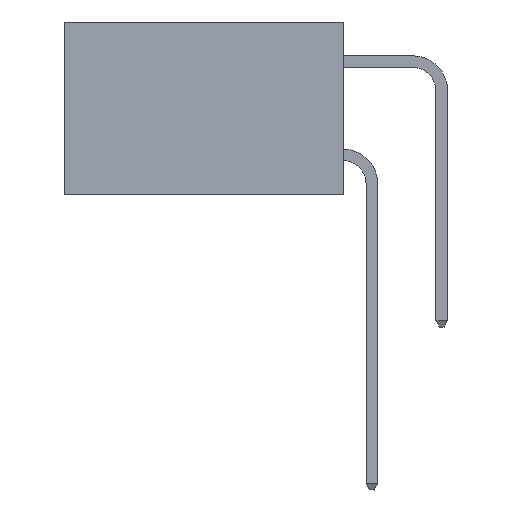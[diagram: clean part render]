
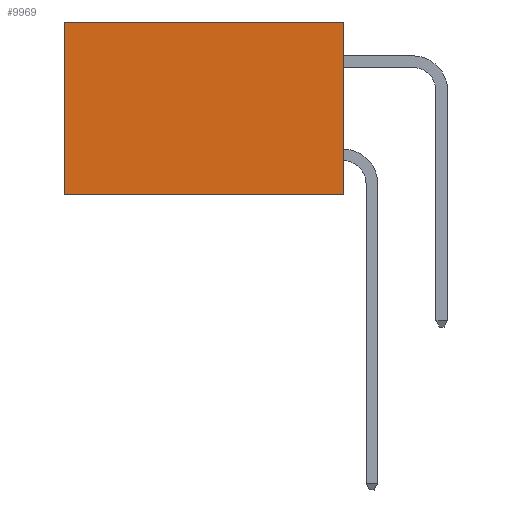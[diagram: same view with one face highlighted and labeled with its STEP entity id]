
A CAD part, left-side view. The second image highlights one B-rep face of the part: STEP entity #9969.
In plain terms, the highlighted planar face has unit normal (-1, 0, 0).
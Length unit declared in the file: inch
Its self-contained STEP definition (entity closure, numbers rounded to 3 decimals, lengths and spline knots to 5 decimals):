
#411 = CARTESIAN_POINT ( 'NONE',  ( 0.298, 0., 0. ) ) ;
#684 = CARTESIAN_POINT ( 'NONE',  ( 0.298, 0., -0.37 ) ) ;
#968 = CARTESIAN_POINT ( 'NONE',  ( 0.298, 0., 0. ) ) ;
#1113 = LINE ( 'NONE', #684, #7513 ) ;
#1353 = ORIENTED_EDGE ( 'NONE', *, *, #10987, .F. ) ;
#1710 = DIRECTION ( 'NONE',  ( 0., 0., -1. ) ) ;
#2029 = ORIENTED_EDGE ( 'NONE', *, *, #10801, .F. ) ;
#2279 = EDGE_CURVE ( 'NONE', #3200, #11761, #5873, .T. ) ;
#3200 = VERTEX_POINT ( 'NONE', #13769 ) ;
#3452 = FACE_OUTER_BOUND ( 'NONE', #10960, .T. ) ;
#3760 = AXIS2_PLACEMENT_3D ( 'NONE', #968, #6488, #12263 ) ;
#3958 = VECTOR ( 'NONE', #9448, 39.37008 ) ;
#5003 = VECTOR ( 'NONE', #1710, 39.37008 ) ;
#5444 = ORIENTED_EDGE ( 'NONE', *, *, #2279, .T. ) ;
#5873 = LINE ( 'NONE', #13036, #5003 ) ;
#6309 = CARTESIAN_POINT ( 'NONE',  ( 0.298, 0., 0. ) ) ;
#6488 = DIRECTION ( 'NONE',  ( 1., 0., 0. ) ) ;
#6939 = CARTESIAN_POINT ( 'NONE',  ( 0.298, 0., -0.37 ) ) ;
#7513 = VECTOR ( 'NONE', #8645, 39.37008 ) ;
#8645 = DIRECTION ( 'NONE',  ( 0., 1., 0. ) ) ;
#9131 = LINE ( 'NONE', #12511, #13186 ) ;
#9262 = ORIENTED_EDGE ( 'NONE', *, *, #10440, .T. ) ;
#9448 = DIRECTION ( 'NONE',  ( 0., 1., 0. ) ) ;
#9969 = ADVANCED_FACE ( 'NONE', ( #3452 ), #10057, .F. ) ;
#10057 = PLANE ( 'NONE',  #3760 ) ;
#10163 = CARTESIAN_POINT ( 'NONE',  ( 0.298, 0.6, -0.37 ) ) ;
#10440 = EDGE_CURVE ( 'NONE', #11594, #3200, #12871, .T. ) ;
#10801 = EDGE_CURVE ( 'NONE', #11594, #14323, #9131, .T. ) ;
#10960 = EDGE_LOOP ( 'NONE', ( #5444, #1353, #2029, #9262 ) ) ;
#10987 = EDGE_CURVE ( 'NONE', #14323, #11761, #1113, .T. ) ;
#11594 = VERTEX_POINT ( 'NONE', #6309 ) ;
#11761 = VERTEX_POINT ( 'NONE', #10163 ) ;
#12263 = DIRECTION ( 'NONE',  ( 0., 0., -1. ) ) ;
#12511 = CARTESIAN_POINT ( 'NONE',  ( 0.298, 0., 0. ) ) ;
#12871 = LINE ( 'NONE', #411, #3958 ) ;
#13036 = CARTESIAN_POINT ( 'NONE',  ( 0.298, 0.6, 0. ) ) ;
#13186 = VECTOR ( 'NONE', #13641, 39.37008 ) ;
#13641 = DIRECTION ( 'NONE',  ( 0., 0., -1. ) ) ;
#13769 = CARTESIAN_POINT ( 'NONE',  ( 0.298, 0.6, 0. ) ) ;
#14323 = VERTEX_POINT ( 'NONE', #6939 ) ;
